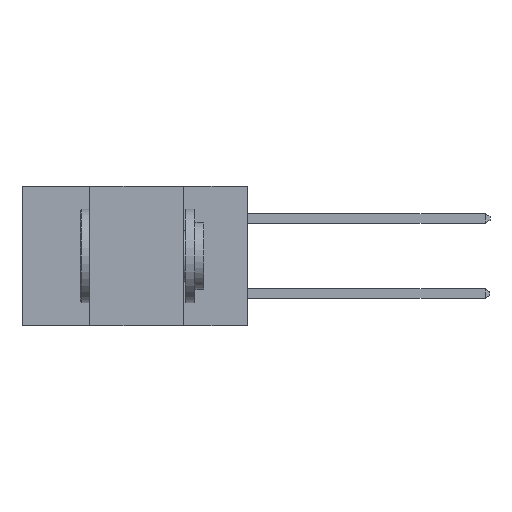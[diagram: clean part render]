
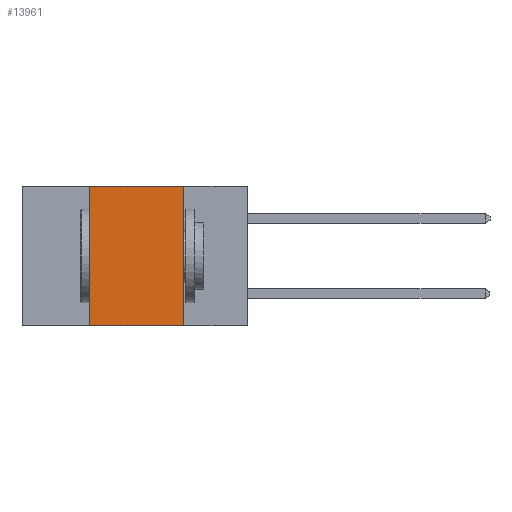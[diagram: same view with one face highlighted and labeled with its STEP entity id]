
A CAD part, left-side view. The second image highlights one B-rep face of the part: STEP entity #13961.
In plain terms, the highlighted planar face has unit normal (-1, 0, 0).
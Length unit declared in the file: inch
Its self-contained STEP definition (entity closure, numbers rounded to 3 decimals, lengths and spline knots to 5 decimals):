
#120 = VECTOR ( 'NONE', #5593, 39.37008 ) ;
#514 = PLANE ( 'NONE',  #9171 ) ;
#742 = EDGE_CURVE ( 'NONE', #2999, #1403, #4015, .T. ) ;
#1403 = VERTEX_POINT ( 'NONE', #2394 ) ;
#2394 = CARTESIAN_POINT ( 'NONE',  ( 0., 0.42, 0. ) ) ;
#2858 = ORIENTED_EDGE ( 'NONE', *, *, #10129, .T. ) ;
#2999 = VERTEX_POINT ( 'NONE', #8736 ) ;
#3041 = LINE ( 'NONE', #6868, #120 ) ;
#3255 = ORIENTED_EDGE ( 'NONE', *, *, #8759, .F. ) ;
#3273 = LINE ( 'NONE', #11546, #11641 ) ;
#3828 = CARTESIAN_POINT ( 'NONE',  ( 0., 0.6, 0. ) ) ;
#4015 = LINE ( 'NONE', #8353, #12293 ) ;
#4692 = VECTOR ( 'NONE', #11718, 39.37008 ) ;
#4936 = DIRECTION ( 'NONE',  ( 0., 0., -1. ) ) ;
#4976 = DIRECTION ( 'NONE',  ( 0., 0., 1. ) ) ;
#5234 = VERTEX_POINT ( 'NONE', #10488 ) ;
#5577 = ORIENTED_EDGE ( 'NONE', *, *, #742, .F. ) ;
#5593 = DIRECTION ( 'NONE',  ( 0., -1., 0. ) ) ;
#6297 = EDGE_CURVE ( 'NONE', #1403, #5234, #3041, .T. ) ;
#6868 = CARTESIAN_POINT ( 'NONE',  ( 0., 0.6, 0. ) ) ;
#8353 = CARTESIAN_POINT ( 'NONE',  ( 0., 0.42, 0. ) ) ;
#8736 = CARTESIAN_POINT ( 'NONE',  ( 0., 0.42, -0.37 ) ) ;
#8759 = EDGE_CURVE ( 'NONE', #5234, #13951, #3273, .T. ) ;
#9171 = AXIS2_PLACEMENT_3D ( 'NONE', #3828, #11461, #4936 ) ;
#10129 = EDGE_CURVE ( 'NONE', #2999, #13951, #12589, .T. ) ;
#10319 = EDGE_LOOP ( 'NONE', ( #3255, #12463, #5577, #2858 ) ) ;
#10418 = CARTESIAN_POINT ( 'NONE',  ( 0., 0.17, -0.37 ) ) ;
#10488 = CARTESIAN_POINT ( 'NONE',  ( 0., 0.17, 0. ) ) ;
#11461 = DIRECTION ( 'NONE',  ( 1., 0., 0. ) ) ;
#11546 = CARTESIAN_POINT ( 'NONE',  ( 0., 0.17, 0. ) ) ;
#11641 = VECTOR ( 'NONE', #13600, 39.37008 ) ;
#11718 = DIRECTION ( 'NONE',  ( 0., -1., 0. ) ) ;
#11794 = CARTESIAN_POINT ( 'NONE',  ( 0., 0.6, -0.37 ) ) ;
#12293 = VECTOR ( 'NONE', #4976, 39.37008 ) ;
#12463 = ORIENTED_EDGE ( 'NONE', *, *, #6297, .F. ) ;
#12571 = FACE_OUTER_BOUND ( 'NONE', #10319, .T. ) ;
#12589 = LINE ( 'NONE', #11794, #4692 ) ;
#13600 = DIRECTION ( 'NONE',  ( 0., 0., -1. ) ) ;
#13951 = VERTEX_POINT ( 'NONE', #10418 ) ;
#13961 = ADVANCED_FACE ( 'NONE', ( #12571 ), #514, .F. ) ;
